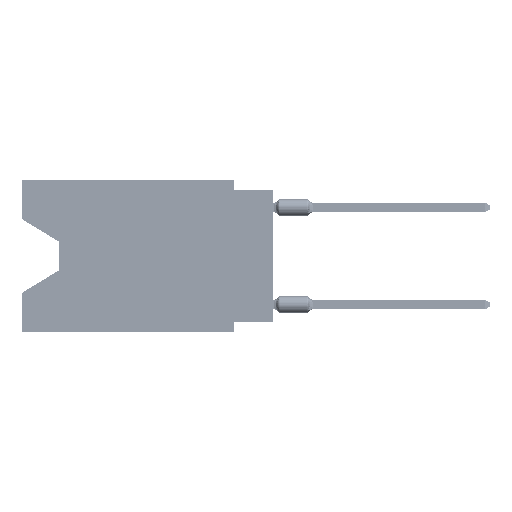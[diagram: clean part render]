
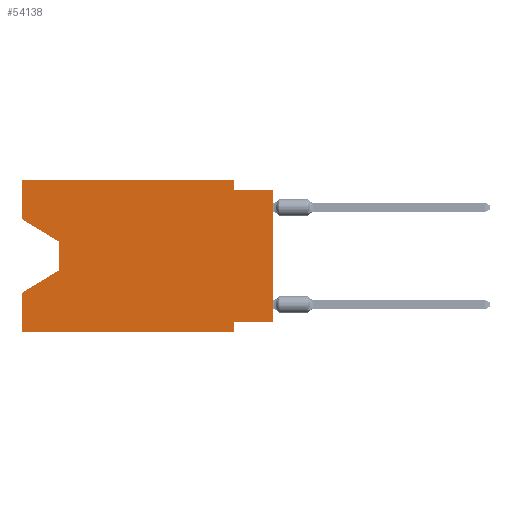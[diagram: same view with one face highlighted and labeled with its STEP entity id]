
A CAD part, left-side view. The second image highlights one B-rep face of the part: STEP entity #54138.
In plain terms, the highlighted planar face has unit normal (-1, 0, 0).
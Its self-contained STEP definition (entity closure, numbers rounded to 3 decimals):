
#443 = VECTOR ( 'NONE', #12814, 1000. ) ;
#929 = CARTESIAN_POINT ( 'NONE',  ( 0., 13.97, -5.893 ) ) ;
#1032 = VERTEX_POINT ( 'NONE', #2277 ) ;
#1259 = EDGE_CURVE ( 'NONE', #55439, #56109, #41829, .T. ) ;
#1382 = PLANE ( 'NONE',  #57914 ) ;
#2277 = CARTESIAN_POINT ( 'NONE',  ( 0., 16.383, 0. ) ) ;
#2365 = EDGE_CURVE ( 'NONE', #8590, #61406, #52211, .T. ) ;
#2820 = CARTESIAN_POINT ( 'NONE',  ( 0., 16.383, -2.546 ) ) ;
#5619 = VERTEX_POINT ( 'NONE', #9551 ) ;
#6218 = LINE ( 'NONE', #28911, #34917 ) ;
#6697 = CARTESIAN_POINT ( 'NONE',  ( 0., 13.97, -4.013 ) ) ;
#6942 = CARTESIAN_POINT ( 'NONE',  ( 0., 2.54, -9.906 ) ) ;
#7366 = EDGE_CURVE ( 'NONE', #23273, #8590, #31439, .T. ) ;
#8590 = VERTEX_POINT ( 'NONE', #6697 ) ;
#9079 = VECTOR ( 'NONE', #57747, 1000. ) ;
#9551 = CARTESIAN_POINT ( 'NONE',  ( 0., 16.383, -7.36 ) ) ;
#10281 = VERTEX_POINT ( 'NONE', #43134 ) ;
#10811 = LINE ( 'NONE', #35056, #9079 ) ;
#11814 = DIRECTION ( 'NONE',  ( 0., -1., 0. ) ) ;
#11903 = DIRECTION ( 'NONE',  ( 0., -1., 0. ) ) ;
#12096 = ORIENTED_EDGE ( 'NONE', *, *, #30211, .F. ) ;
#12365 = ORIENTED_EDGE ( 'NONE', *, *, #33666, .F. ) ;
#12814 = DIRECTION ( 'NONE',  ( 0., 0.855, -0.519 ) ) ;
#12969 = VECTOR ( 'NONE', #11814, 1000. ) ;
#15170 = DIRECTION ( 'NONE',  ( 0., 1., 0. ) ) ;
#15815 = EDGE_CURVE ( 'NONE', #61406, #5619, #71305, .T. ) ;
#16068 = DIRECTION ( 'NONE',  ( 0., 0., -1. ) ) ;
#16827 = LINE ( 'NONE', #58760, #35261 ) ;
#17585 = CARTESIAN_POINT ( 'NONE',  ( 0., 16.383, -9.906 ) ) ;
#17667 = LINE ( 'NONE', #64614, #32337 ) ;
#17745 = DIRECTION ( 'NONE',  ( 0., 0., 1. ) ) ;
#18594 = CARTESIAN_POINT ( 'NONE',  ( 0., 13.97, -5.893 ) ) ;
#20185 = CARTESIAN_POINT ( 'NONE',  ( 0., 16.383, -9.906 ) ) ;
#21448 = EDGE_CURVE ( 'NONE', #37957, #32716, #24486, .T. ) ;
#22083 = DIRECTION ( 'NONE',  ( 0., 0., -1. ) ) ;
#23273 = VERTEX_POINT ( 'NONE', #2820 ) ;
#24486 = LINE ( 'NONE', #71416, #50264 ) ;
#26032 = ORIENTED_EDGE ( 'NONE', *, *, #7366, .T. ) ;
#28052 = ORIENTED_EDGE ( 'NONE', *, *, #38755, .F. ) ;
#28911 = CARTESIAN_POINT ( 'NONE',  ( 0., 16.383, 0. ) ) ;
#30211 = EDGE_CURVE ( 'NONE', #37957, #10281, #72919, .T. ) ;
#30349 = ORIENTED_EDGE ( 'NONE', *, *, #2365, .T. ) ;
#30611 = FACE_OUTER_BOUND ( 'NONE', #37363, .T. ) ;
#30643 = VECTOR ( 'NONE', #60680, 1000. ) ;
#31439 = LINE ( 'NONE', #55675, #30643 ) ;
#32337 = VECTOR ( 'NONE', #11903, 1000. ) ;
#32716 = VERTEX_POINT ( 'NONE', #62378 ) ;
#32827 = ORIENTED_EDGE ( 'NONE', *, *, #1259, .T. ) ;
#33060 = CARTESIAN_POINT ( 'NONE',  ( 0., 2.54, 0. ) ) ;
#33666 = EDGE_CURVE ( 'NONE', #10281, #56109, #64385, .T. ) ;
#34917 = VECTOR ( 'NONE', #17745, 1000. ) ;
#35056 = CARTESIAN_POINT ( 'NONE',  ( 0., 16.383, 0. ) ) ;
#35261 = VECTOR ( 'NONE', #56208, 1000. ) ;
#37363 = EDGE_LOOP ( 'NONE', ( #26032, #30349, #74505, #44274, #32827, #12365, #12096, #41382, #44438, #51182, #70572, #28052 ) ) ;
#37719 = LINE ( 'NONE', #33060, #56953 ) ;
#37957 = VERTEX_POINT ( 'NONE', #69473 ) ;
#38755 = EDGE_CURVE ( 'NONE', #23273, #1032, #10811, .T. ) ;
#39036 = EDGE_CURVE ( 'NONE', #50366, #52880, #37719, .T. ) ;
#40304 = CARTESIAN_POINT ( 'NONE',  ( 0., 13.97, -4.013 ) ) ;
#41382 = ORIENTED_EDGE ( 'NONE', *, *, #21448, .T. ) ;
#41829 = LINE ( 'NONE', #17585, #12969 ) ;
#42538 = CARTESIAN_POINT ( 'NONE',  ( 0., 16.383, 0. ) ) ;
#42896 = CARTESIAN_POINT ( 'NONE',  ( 0., 2.54, -0.635 ) ) ;
#43134 = CARTESIAN_POINT ( 'NONE',  ( 0., 2.54, -9.271 ) ) ;
#44274 = ORIENTED_EDGE ( 'NONE', *, *, #63159, .F. ) ;
#44438 = ORIENTED_EDGE ( 'NONE', *, *, #70042, .F. ) ;
#45012 = VECTOR ( 'NONE', #15170, 1000. ) ;
#47989 = CARTESIAN_POINT ( 'NONE',  ( 0., 2.54, 0. ) ) ;
#49059 = DIRECTION ( 'NONE',  ( 1., 0., 0. ) ) ;
#50264 = VECTOR ( 'NONE', #64874, 1000. ) ;
#50366 = VERTEX_POINT ( 'NONE', #47989 ) ;
#51182 = ORIENTED_EDGE ( 'NONE', *, *, #39036, .F. ) ;
#52211 = LINE ( 'NONE', #40304, #74523 ) ;
#52880 = VERTEX_POINT ( 'NONE', #42896 ) ;
#53319 = DIRECTION ( 'NONE',  ( 0., 0., -1. ) ) ;
#54138 = ADVANCED_FACE ( 'NONE', ( #30611 ), #1382, .F. ) ;
#55439 = VERTEX_POINT ( 'NONE', #20185 ) ;
#55675 = CARTESIAN_POINT ( 'NONE',  ( 0., 16.383, -2.546 ) ) ;
#56109 = VERTEX_POINT ( 'NONE', #6942 ) ;
#56208 = DIRECTION ( 'NONE',  ( 0., -1., 0. ) ) ;
#56953 = VECTOR ( 'NONE', #67700, 1000. ) ;
#57747 = DIRECTION ( 'NONE',  ( 0., 0., 1. ) ) ;
#57914 = AXIS2_PLACEMENT_3D ( 'NONE', #42538, #49059, #53319 ) ;
#58613 = CARTESIAN_POINT ( 'NONE',  ( 0., 2.54, -9.906 ) ) ;
#58760 = CARTESIAN_POINT ( 'NONE',  ( 0., 0., -0.635 ) ) ;
#60680 = DIRECTION ( 'NONE',  ( 0., -0.855, -0.519 ) ) ;
#61406 = VERTEX_POINT ( 'NONE', #929 ) ;
#62299 = EDGE_CURVE ( 'NONE', #1032, #50366, #17667, .T. ) ;
#62378 = CARTESIAN_POINT ( 'NONE',  ( 0., 0., -0.635 ) ) ;
#63159 = EDGE_CURVE ( 'NONE', #55439, #5619, #6218, .T. ) ;
#64385 = LINE ( 'NONE', #58613, #72585 ) ;
#64614 = CARTESIAN_POINT ( 'NONE',  ( 0., 16.383, 0. ) ) ;
#64874 = DIRECTION ( 'NONE',  ( 0., 0., 1. ) ) ;
#67700 = DIRECTION ( 'NONE',  ( 0., 0., -1. ) ) ;
#67905 = CARTESIAN_POINT ( 'NONE',  ( 0., 0., -9.271 ) ) ;
#69473 = CARTESIAN_POINT ( 'NONE',  ( 0., 0., -9.271 ) ) ;
#70042 = EDGE_CURVE ( 'NONE', #52880, #32716, #16827, .T. ) ;
#70572 = ORIENTED_EDGE ( 'NONE', *, *, #62299, .F. ) ;
#71305 = LINE ( 'NONE', #18594, #443 ) ;
#71416 = CARTESIAN_POINT ( 'NONE',  ( 0., 0., 0. ) ) ;
#72585 = VECTOR ( 'NONE', #22083, 1000. ) ;
#72919 = LINE ( 'NONE', #67905, #45012 ) ;
#74505 = ORIENTED_EDGE ( 'NONE', *, *, #15815, .T. ) ;
#74523 = VECTOR ( 'NONE', #16068, 1000. ) ;
